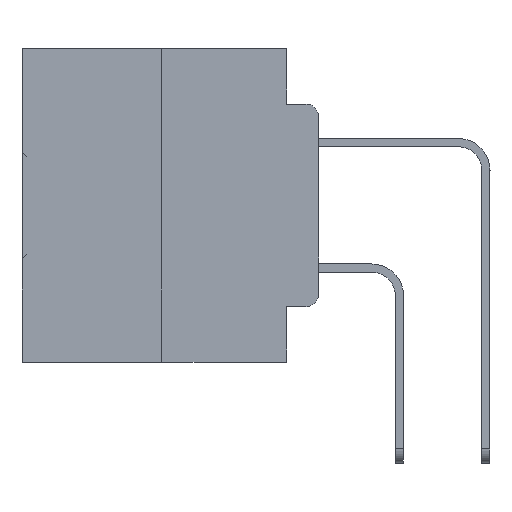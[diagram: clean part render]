
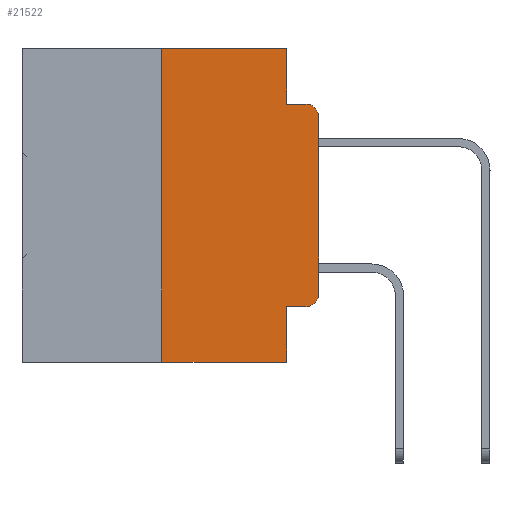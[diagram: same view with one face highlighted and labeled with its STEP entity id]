
A CAD part, left-side view. The second image highlights one B-rep face of the part: STEP entity #21522.
In plain terms, the highlighted planar face has unit normal (-1, 0, 0).
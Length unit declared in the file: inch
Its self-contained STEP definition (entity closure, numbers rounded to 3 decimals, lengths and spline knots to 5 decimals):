
#16 = VECTOR ( 'NONE', #14033, 39.37008 ) ;
#137 = CARTESIAN_POINT ( 'NONE',  ( 0., 0.02, -0.4115 ) ) ;
#582 = LINE ( 'NONE', #10990, #17398 ) ;
#2132 = CARTESIAN_POINT ( 'NONE',  ( 0., 0.051, -0.0885 ) ) ;
#2458 = EDGE_CURVE ( 'NONE', #31801, #4803, #34819, .T. ) ;
#3023 = EDGE_CURVE ( 'NONE', #6787, #24477, #27608, .T. ) ;
#3197 = FACE_OUTER_BOUND ( 'NONE', #23031, .T. ) ;
#3254 = CARTESIAN_POINT ( 'NONE',  ( 0., 0.02, -0.0885 ) ) ;
#3548 = ORIENTED_EDGE ( 'NONE', *, *, #12492, .F. ) ;
#3690 = DIRECTION ( 'NONE',  ( 0., 0., -1. ) ) ;
#4393 = ORIENTED_EDGE ( 'NONE', *, *, #15250, .T. ) ;
#4803 = VERTEX_POINT ( 'NONE', #8537 ) ;
#4871 = LINE ( 'NONE', #32102, #10621 ) ;
#5124 = ORIENTED_EDGE ( 'NONE', *, *, #31963, .T. ) ;
#5163 = CARTESIAN_POINT ( 'NONE',  ( 0., 0., -0.1085 ) ) ;
#5355 = DIRECTION ( 'NONE',  ( 0., 0., -1. ) ) ;
#5625 = VECTOR ( 'NONE', #25294, 39.37008 ) ;
#5702 = EDGE_CURVE ( 'NONE', #4803, #29885, #28444, .T. ) ;
#5897 = CARTESIAN_POINT ( 'NONE',  ( 0., 0.051, -0.5 ) ) ;
#5982 = EDGE_CURVE ( 'NONE', #24477, #18972, #33566, .T. ) ;
#6315 = ORIENTED_EDGE ( 'NONE', *, *, #28553, .F. ) ;
#6787 = VERTEX_POINT ( 'NONE', #137 ) ;
#7582 = ORIENTED_EDGE ( 'NONE', *, *, #8918, .T. ) ;
#8537 = CARTESIAN_POINT ( 'NONE',  ( 0., 0.25, 0. ) ) ;
#8560 = PLANE ( 'NONE',  #21910 ) ;
#8728 = CARTESIAN_POINT ( 'NONE',  ( 0., 0.02, -0.3915 ) ) ;
#8918 = EDGE_CURVE ( 'NONE', #32555, #6787, #582, .T. ) ;
#10264 = ORIENTED_EDGE ( 'NONE', *, *, #3023, .T. ) ;
#10621 = VECTOR ( 'NONE', #26907, 39.37008 ) ;
#10990 = CARTESIAN_POINT ( 'NONE',  ( 0., 0.051, -0.4115 ) ) ;
#11043 = CARTESIAN_POINT ( 'NONE',  ( 0., 0.473, -0.5 ) ) ;
#11236 = LINE ( 'NONE', #11043, #27250 ) ;
#11580 = AXIS2_PLACEMENT_3D ( 'NONE', #8728, #13772, #3690 ) ;
#11774 = VERTEX_POINT ( 'NONE', #5897 ) ;
#11855 = VECTOR ( 'NONE', #24432, 39.37008 ) ;
#12492 = EDGE_CURVE ( 'NONE', #27807, #34374, #16704, .T. ) ;
#12793 = ORIENTED_EDGE ( 'NONE', *, *, #22388, .F. ) ;
#12869 = CARTESIAN_POINT ( 'NONE',  ( 0., 0.25, -0.5 ) ) ;
#13772 = DIRECTION ( 'NONE',  ( -1., 0., 0. ) ) ;
#14001 = ORIENTED_EDGE ( 'NONE', *, *, #2458, .F. ) ;
#14033 = DIRECTION ( 'NONE',  ( 0., -1., 0. ) ) ;
#14126 = CARTESIAN_POINT ( 'NONE',  ( 0., 0.473, 0. ) ) ;
#14811 = CARTESIAN_POINT ( 'NONE',  ( 0., 0.473, 0. ) ) ;
#15250 = EDGE_CURVE ( 'NONE', #18972, #34374, #19043, .T. ) ;
#16179 = AXIS2_PLACEMENT_3D ( 'NONE', #29657, #35220, #30350 ) ;
#16704 = LINE ( 'NONE', #21911, #16 ) ;
#17398 = VECTOR ( 'NONE', #33576, 39.37008 ) ;
#18874 = ORIENTED_EDGE ( 'NONE', *, *, #5702, .F. ) ;
#18972 = VERTEX_POINT ( 'NONE', #5163 ) ;
#19043 = CIRCLE ( 'NONE', #16179, 0.02 ) ;
#19492 = DIRECTION ( 'NONE',  ( 1., 0., 0. ) ) ;
#19581 = ORIENTED_EDGE ( 'NONE', *, *, #5982, .T. ) ;
#21522 = ADVANCED_FACE ( 'NONE', ( #3197 ), #8560, .F. ) ;
#21842 = CARTESIAN_POINT ( 'NONE',  ( 0., 0., -0.3915 ) ) ;
#21910 = AXIS2_PLACEMENT_3D ( 'NONE', #14126, #19492, #5355 ) ;
#21911 = CARTESIAN_POINT ( 'NONE',  ( 0., 0.051, -0.0885 ) ) ;
#22388 = EDGE_CURVE ( 'NONE', #32555, #11774, #35263, .T. ) ;
#23031 = EDGE_LOOP ( 'NONE', ( #19581, #4393, #3548, #6315, #18874, #14001, #5124, #12793, #7582, #10264 ) ) ;
#23702 = CARTESIAN_POINT ( 'NONE',  ( 0., 0.25, 0. ) ) ;
#24432 = DIRECTION ( 'NONE',  ( 0., 0., 1. ) ) ;
#24477 = VERTEX_POINT ( 'NONE', #21842 ) ;
#24519 = DIRECTION ( 'NONE',  ( 0., -1., 0. ) ) ;
#25294 = DIRECTION ( 'NONE',  ( 0., 0., 1. ) ) ;
#25715 = CARTESIAN_POINT ( 'NONE',  ( 0., 0.051, 0. ) ) ;
#26907 = DIRECTION ( 'NONE',  ( 0., 0., -1. ) ) ;
#27250 = VECTOR ( 'NONE', #24519, 39.37008 ) ;
#27608 = CIRCLE ( 'NONE', #11580, 0.02 ) ;
#27694 = VECTOR ( 'NONE', #29153, 39.37008 ) ;
#27807 = VERTEX_POINT ( 'NONE', #2132 ) ;
#28444 = LINE ( 'NONE', #14811, #32534 ) ;
#28553 = EDGE_CURVE ( 'NONE', #29885, #27807, #4871, .T. ) ;
#29153 = DIRECTION ( 'NONE',  ( 0., 0., -1. ) ) ;
#29657 = CARTESIAN_POINT ( 'NONE',  ( 0., 0.02, -0.1085 ) ) ;
#29862 = CARTESIAN_POINT ( 'NONE',  ( 0., 0.051, 0. ) ) ;
#29885 = VERTEX_POINT ( 'NONE', #25715 ) ;
#30350 = DIRECTION ( 'NONE',  ( 0., 0., -1. ) ) ;
#30703 = CARTESIAN_POINT ( 'NONE',  ( 0., 0., 0. ) ) ;
#31318 = DIRECTION ( 'NONE',  ( 0., -1., 0. ) ) ;
#31801 = VERTEX_POINT ( 'NONE', #12869 ) ;
#31963 = EDGE_CURVE ( 'NONE', #31801, #11774, #11236, .T. ) ;
#32102 = CARTESIAN_POINT ( 'NONE',  ( 0., 0.051, 0. ) ) ;
#32534 = VECTOR ( 'NONE', #31318, 39.37008 ) ;
#32555 = VERTEX_POINT ( 'NONE', #33922 ) ;
#33566 = LINE ( 'NONE', #30703, #5625 ) ;
#33576 = DIRECTION ( 'NONE',  ( 0., -1., 0. ) ) ;
#33922 = CARTESIAN_POINT ( 'NONE',  ( 0., 0.051, -0.4115 ) ) ;
#34374 = VERTEX_POINT ( 'NONE', #3254 ) ;
#34819 = LINE ( 'NONE', #23702, #11855 ) ;
#35220 = DIRECTION ( 'NONE',  ( -1., 0., 0. ) ) ;
#35263 = LINE ( 'NONE', #29862, #27694 ) ;
